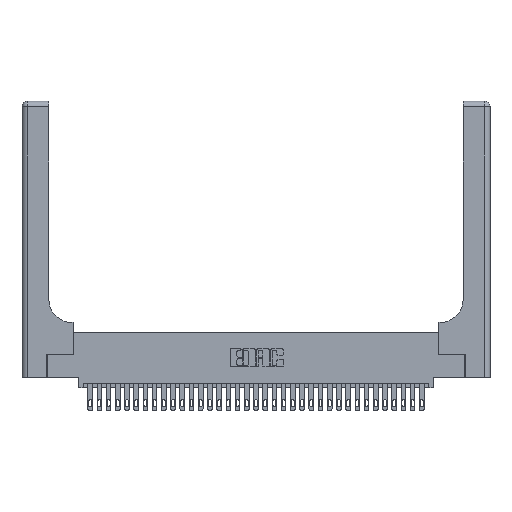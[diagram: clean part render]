
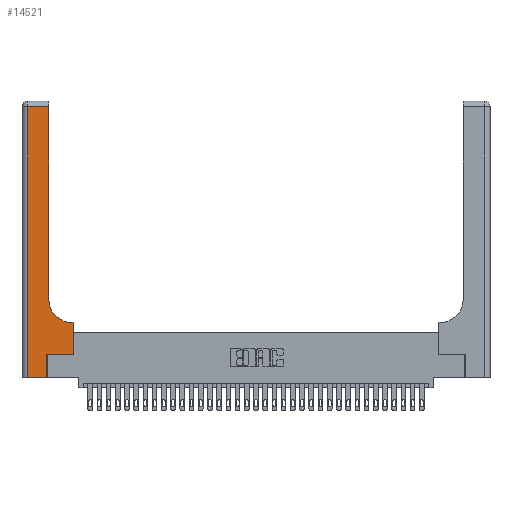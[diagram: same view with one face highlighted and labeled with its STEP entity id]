
A CAD part, top view. The second image highlights one B-rep face of the part: STEP entity #14521.
In plain terms, the highlighted planar face has unit normal (0, 0, 1).
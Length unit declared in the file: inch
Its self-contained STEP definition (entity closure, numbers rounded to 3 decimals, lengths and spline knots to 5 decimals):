
#23 = DIRECTION ( 'NONE',  ( 0., 0., -1. ) ) ;
#24 = LINE ( 'NONE', #11122, #22007 ) ;
#37 = CIRCLE ( 'NONE', #22397, 0.25 ) ;
#1033 = CARTESIAN_POINT ( 'NONE',  ( 0., 3., 0.37 ) ) ;
#1866 = VECTOR ( 'NONE', #3293, 39.37008 ) ;
#2474 = VERTEX_POINT ( 'NONE', #20139 ) ;
#2671 = CARTESIAN_POINT ( 'NONE',  ( 0.5415, 0.85, 0.37 ) ) ;
#2781 = DIRECTION ( 'NONE',  ( 1., 0., 0. ) ) ;
#3252 = EDGE_CURVE ( 'NONE', #28568, #13570, #33375, .T. ) ;
#3293 = DIRECTION ( 'NONE',  ( 1., 0., 0. ) ) ;
#4068 = DIRECTION ( 'NONE',  ( 0., 1., 0. ) ) ;
#4916 = ORIENTED_EDGE ( 'NONE', *, *, #24780, .T. ) ;
#5186 = EDGE_CURVE ( 'NONE', #21064, #28568, #11676, .T. ) ;
#5363 = ORIENTED_EDGE ( 'NONE', *, *, #21091, .T. ) ;
#6077 = VERTEX_POINT ( 'NONE', #15059 ) ;
#6745 = CARTESIAN_POINT ( 'NONE',  ( 0.5585, 0.6, 0.37 ) ) ;
#7009 = DIRECTION ( 'NONE',  ( 0., 0., -1. ) ) ;
#7049 = VECTOR ( 'NONE', #23292, 39.37008 ) ;
#7667 = EDGE_CURVE ( 'NONE', #33750, #21064, #34243, .T. ) ;
#8201 = CARTESIAN_POINT ( 'NONE',  ( 0.269, 0., 0.37 ) ) ;
#8270 = ORIENTED_EDGE ( 'NONE', *, *, #22550, .T. ) ;
#9244 = VECTOR ( 'NONE', #25935, 39.37008 ) ;
#9457 = CARTESIAN_POINT ( 'NONE',  ( 0.2915, 0.6, 0.37 ) ) ;
#10126 = VERTEX_POINT ( 'NONE', #12067 ) ;
#10888 = ORIENTED_EDGE ( 'NONE', *, *, #15226, .T. ) ;
#11122 = CARTESIAN_POINT ( 'NONE',  ( 0.2915, 3., 0.37 ) ) ;
#11676 = LINE ( 'NONE', #29234, #13779 ) ;
#12067 = CARTESIAN_POINT ( 'NONE',  ( 0.5415, 0.6, 0.37 ) ) ;
#12610 = ORIENTED_EDGE ( 'NONE', *, *, #20052, .T. ) ;
#13570 = VERTEX_POINT ( 'NONE', #6745 ) ;
#13779 = VECTOR ( 'NONE', #15444, 39.37008 ) ;
#14367 = VECTOR ( 'NONE', #23922, 39.37008 ) ;
#14521 = ADVANCED_FACE ( 'NONE', ( #26002 ), #16567, .F. ) ;
#15059 = CARTESIAN_POINT ( 'NONE',  ( 0.06, 2.94, 0.37 ) ) ;
#15226 = EDGE_CURVE ( 'NONE', #26729, #33750, #32695, .T. ) ;
#15444 = DIRECTION ( 'NONE',  ( 1., 0., 0. ) ) ;
#15729 = CARTESIAN_POINT ( 'NONE',  ( 0., 2.94, 0.37 ) ) ;
#16264 = CARTESIAN_POINT ( 'NONE',  ( 0.269, 0.25, 0.37 ) ) ;
#16567 = PLANE ( 'NONE',  #18215 ) ;
#16771 = EDGE_CURVE ( 'NONE', #26762, #2474, #24, .T. ) ;
#16863 = CARTESIAN_POINT ( 'NONE',  ( 0., 0., 0.37 ) ) ;
#17193 = ORIENTED_EDGE ( 'NONE', *, *, #16771, .T. ) ;
#17322 = ORIENTED_EDGE ( 'NONE', *, *, #3252, .T. ) ;
#17384 = CARTESIAN_POINT ( 'NONE',  ( 0.5585, 0.25, 0.37 ) ) ;
#17915 = ORIENTED_EDGE ( 'NONE', *, *, #7667, .T. ) ;
#18080 = VECTOR ( 'NONE', #26310, 39.37008 ) ;
#18215 = AXIS2_PLACEMENT_3D ( 'NONE', #1033, #7009, #19954 ) ;
#19954 = DIRECTION ( 'NONE',  ( -1., 0., 0. ) ) ;
#20052 = EDGE_CURVE ( 'NONE', #2474, #6077, #32413, .T. ) ;
#20139 = CARTESIAN_POINT ( 'NONE',  ( 0.2915, 2.94, 0.37 ) ) ;
#20808 = CARTESIAN_POINT ( 'NONE',  ( 0.06, 0., 0.37 ) ) ;
#20951 = CARTESIAN_POINT ( 'NONE',  ( 0.5585, 0.25, 0.37 ) ) ;
#21064 = VERTEX_POINT ( 'NONE', #16264 ) ;
#21091 = EDGE_CURVE ( 'NONE', #10126, #26762, #37, .T. ) ;
#22007 = VECTOR ( 'NONE', #22334, 39.37008 ) ;
#22334 = DIRECTION ( 'NONE',  ( 0., 1., 0. ) ) ;
#22397 = AXIS2_PLACEMENT_3D ( 'NONE', #2671, #23, #2781 ) ;
#22407 = VECTOR ( 'NONE', #4068, 39.37008 ) ;
#22473 = ORIENTED_EDGE ( 'NONE', *, *, #5186, .T. ) ;
#22550 = EDGE_CURVE ( 'NONE', #6077, #26729, #29571, .T. ) ;
#23292 = DIRECTION ( 'NONE',  ( -1., 0., 0. ) ) ;
#23922 = DIRECTION ( 'NONE',  ( 0., 1., 0. ) ) ;
#24780 = EDGE_CURVE ( 'NONE', #13570, #10126, #32778, .T. ) ;
#25571 = CARTESIAN_POINT ( 'NONE',  ( 0.06, 3., 0.37 ) ) ;
#25935 = DIRECTION ( 'NONE',  ( 0., -1., 0. ) ) ;
#26002 = FACE_OUTER_BOUND ( 'NONE', #27837, .T. ) ;
#26310 = DIRECTION ( 'NONE',  ( -1., 0., 0. ) ) ;
#26541 = CARTESIAN_POINT ( 'NONE',  ( 0.2915, 0.85, 0.37 ) ) ;
#26729 = VERTEX_POINT ( 'NONE', #20808 ) ;
#26762 = VERTEX_POINT ( 'NONE', #26541 ) ;
#27837 = EDGE_LOOP ( 'NONE', ( #17193, #12610, #8270, #10888, #17915, #22473, #17322, #4916, #5363 ) ) ;
#28568 = VERTEX_POINT ( 'NONE', #17384 ) ;
#29234 = CARTESIAN_POINT ( 'NONE',  ( 0.269, 0.25, 0.37 ) ) ;
#29571 = LINE ( 'NONE', #25571, #9244 ) ;
#31107 = CARTESIAN_POINT ( 'NONE',  ( 0.269, 0., 0.37 ) ) ;
#32413 = LINE ( 'NONE', #15729, #18080 ) ;
#32695 = LINE ( 'NONE', #16863, #1866 ) ;
#32778 = LINE ( 'NONE', #9457, #7049 ) ;
#33375 = LINE ( 'NONE', #20951, #14367 ) ;
#33750 = VERTEX_POINT ( 'NONE', #8201 ) ;
#34243 = LINE ( 'NONE', #31107, #22407 ) ;
